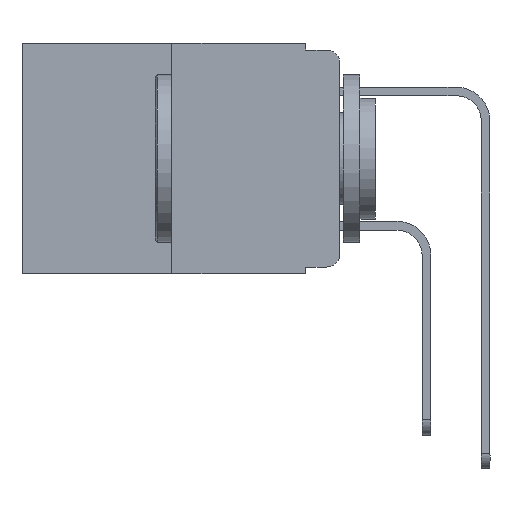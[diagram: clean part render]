
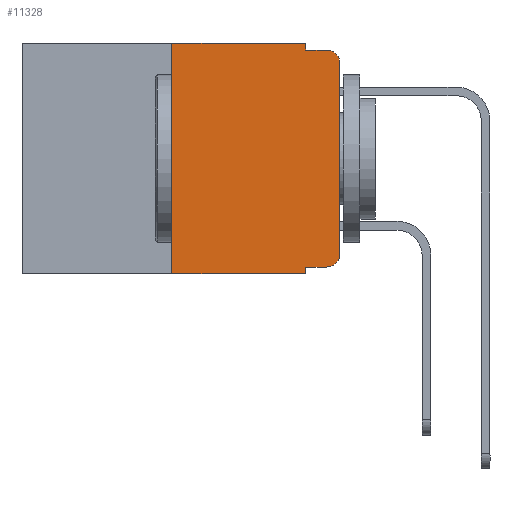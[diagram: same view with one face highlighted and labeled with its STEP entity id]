
A CAD part, left-side view. The second image highlights one B-rep face of the part: STEP entity #11328.
In plain terms, the highlighted planar face has unit normal (-1, 0, 0).
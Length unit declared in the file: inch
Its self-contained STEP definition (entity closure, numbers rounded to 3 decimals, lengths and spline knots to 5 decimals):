
#223 = AXIS2_PLACEMENT_3D ( 'NONE', #868, #13849, #3503 ) ;
#466 = EDGE_CURVE ( 'NONE', #8250, #16321, #9810, .T. ) ;
#662 = VERTEX_POINT ( 'NONE', #15351 ) ;
#868 = CARTESIAN_POINT ( 'NONE',  ( 0., 0.473, 0. ) ) ;
#1237 = DIRECTION ( 'NONE',  ( 0., 0., -1. ) ) ;
#1440 = VERTEX_POINT ( 'NONE', #16338 ) ;
#1577 = DIRECTION ( 'NONE',  ( 0., -1., 0. ) ) ;
#1847 = CARTESIAN_POINT ( 'NONE',  ( 0., 0.051, -0.343 ) ) ;
#1864 = CIRCLE ( 'NONE', #2945, 0.02 ) ;
#2131 = CARTESIAN_POINT ( 'NONE',  ( 0., 0., 0. ) ) ;
#2136 = VERTEX_POINT ( 'NONE', #7594 ) ;
#2229 = CARTESIAN_POINT ( 'NONE',  ( 0., 0.473, 0. ) ) ;
#2482 = DIRECTION ( 'NONE',  ( -1., 0., 0. ) ) ;
#2513 = CARTESIAN_POINT ( 'NONE',  ( 0., 0.02, -0.333 ) ) ;
#2811 = EDGE_CURVE ( 'NONE', #7481, #9059, #2869, .T. ) ;
#2869 = LINE ( 'NONE', #9188, #7181 ) ;
#2945 = AXIS2_PLACEMENT_3D ( 'NONE', #7443, #12659, #11380 ) ;
#3161 = VECTOR ( 'NONE', #6323, 39.37008 ) ;
#3177 = CARTESIAN_POINT ( 'NONE',  ( 0., 0.473, -0.343 ) ) ;
#3304 = ORIENTED_EDGE ( 'NONE', *, *, #466, .T. ) ;
#3503 = DIRECTION ( 'NONE',  ( 0., 0., -1. ) ) ;
#3561 = EDGE_CURVE ( 'NONE', #9451, #8250, #3597, .T. ) ;
#3597 = CIRCLE ( 'NONE', #4415, 0.02 ) ;
#3676 = PLANE ( 'NONE',  #223 ) ;
#3823 = VECTOR ( 'NONE', #1577, 39.37008 ) ;
#3964 = VECTOR ( 'NONE', #7245, 39.37008 ) ;
#4415 = AXIS2_PLACEMENT_3D ( 'NONE', #4936, #2482, #14090 ) ;
#4618 = VERTEX_POINT ( 'NONE', #13183 ) ;
#4823 = ORIENTED_EDGE ( 'NONE', *, *, #9868, .T. ) ;
#4837 = ORIENTED_EDGE ( 'NONE', *, *, #9538, .F. ) ;
#4936 = CARTESIAN_POINT ( 'NONE',  ( 0., 0.02, -0.313 ) ) ;
#4947 = EDGE_CURVE ( 'NONE', #1440, #2136, #16865, .T. ) ;
#5548 = ORIENTED_EDGE ( 'NONE', *, *, #2811, .F. ) ;
#6323 = DIRECTION ( 'NONE',  ( 0., -1., 0. ) ) ;
#7181 = VECTOR ( 'NONE', #12099, 39.37008 ) ;
#7245 = DIRECTION ( 'NONE',  ( 0., 0., 1. ) ) ;
#7443 = CARTESIAN_POINT ( 'NONE',  ( 0., 0.02, -0.03 ) ) ;
#7476 = CARTESIAN_POINT ( 'NONE',  ( 0., 0.051, -0.333 ) ) ;
#7481 = VERTEX_POINT ( 'NONE', #7476 ) ;
#7539 = VECTOR ( 'NONE', #11385, 39.37008 ) ;
#7594 = CARTESIAN_POINT ( 'NONE',  ( 0., 0.25, 0. ) ) ;
#8077 = ORIENTED_EDGE ( 'NONE', *, *, #11386, .T. ) ;
#8250 = VERTEX_POINT ( 'NONE', #14632 ) ;
#8394 = LINE ( 'NONE', #13427, #3823 ) ;
#8482 = VECTOR ( 'NONE', #14196, 39.37008 ) ;
#8981 = CARTESIAN_POINT ( 'NONE',  ( 0., 0.051, -0.333 ) ) ;
#9059 = VERTEX_POINT ( 'NONE', #1847 ) ;
#9102 = ORIENTED_EDGE ( 'NONE', *, *, #12095, .F. ) ;
#9188 = CARTESIAN_POINT ( 'NONE',  ( 0., 0.051, 0. ) ) ;
#9303 = VERTEX_POINT ( 'NONE', #15065 ) ;
#9451 = VERTEX_POINT ( 'NONE', #2513 ) ;
#9538 = EDGE_CURVE ( 'NONE', #662, #9303, #8394, .T. ) ;
#9810 = LINE ( 'NONE', #2131, #3964 ) ;
#9831 = ORIENTED_EDGE ( 'NONE', *, *, #14670, .T. ) ;
#9868 = EDGE_CURVE ( 'NONE', #7481, #9451, #10268, .T. ) ;
#10075 = LINE ( 'NONE', #2229, #3161 ) ;
#10268 = LINE ( 'NONE', #8981, #8482 ) ;
#10976 = ORIENTED_EDGE ( 'NONE', *, *, #3561, .T. ) ;
#11049 = DIRECTION ( 'NONE',  ( 0., -1., 0. ) ) ;
#11328 = ADVANCED_FACE ( 'NONE', ( #16510 ), #3676, .F. ) ;
#11380 = DIRECTION ( 'NONE',  ( 0., 0., -1. ) ) ;
#11385 = DIRECTION ( 'NONE',  ( 0., 0., 1. ) ) ;
#11386 = EDGE_CURVE ( 'NONE', #16321, #9303, #1864, .T. ) ;
#11579 = CARTESIAN_POINT ( 'NONE',  ( 0., 0., -0.03 ) ) ;
#11655 = CARTESIAN_POINT ( 'NONE',  ( 0., 0.051, 0. ) ) ;
#12095 = EDGE_CURVE ( 'NONE', #4618, #662, #15406, .T. ) ;
#12099 = DIRECTION ( 'NONE',  ( 0., 0., -1. ) ) ;
#12659 = DIRECTION ( 'NONE',  ( -1., 0., 0. ) ) ;
#13141 = VECTOR ( 'NONE', #1237, 39.37008 ) ;
#13183 = CARTESIAN_POINT ( 'NONE',  ( 0., 0.051, 0. ) ) ;
#13197 = ORIENTED_EDGE ( 'NONE', *, *, #16644, .F. ) ;
#13427 = CARTESIAN_POINT ( 'NONE',  ( 0., 0.051, -0.01 ) ) ;
#13849 = DIRECTION ( 'NONE',  ( 1., 0., 0. ) ) ;
#13944 = CARTESIAN_POINT ( 'NONE',  ( 0., 0.25, 0. ) ) ;
#14090 = DIRECTION ( 'NONE',  ( 0., 0., -1. ) ) ;
#14094 = ORIENTED_EDGE ( 'NONE', *, *, #4947, .F. ) ;
#14196 = DIRECTION ( 'NONE',  ( 0., -1., 0. ) ) ;
#14589 = VECTOR ( 'NONE', #11049, 39.37008 ) ;
#14632 = CARTESIAN_POINT ( 'NONE',  ( 0., 0., -0.313 ) ) ;
#14670 = EDGE_CURVE ( 'NONE', #1440, #9059, #14885, .T. ) ;
#14885 = LINE ( 'NONE', #3177, #14589 ) ;
#15065 = CARTESIAN_POINT ( 'NONE',  ( 0., 0.02, -0.01 ) ) ;
#15351 = CARTESIAN_POINT ( 'NONE',  ( 0., 0.051, -0.01 ) ) ;
#15406 = LINE ( 'NONE', #11655, #13141 ) ;
#16099 = EDGE_LOOP ( 'NONE', ( #3304, #8077, #4837, #9102, #13197, #14094, #9831, #5548, #4823, #10976 ) ) ;
#16321 = VERTEX_POINT ( 'NONE', #11579 ) ;
#16338 = CARTESIAN_POINT ( 'NONE',  ( 0., 0.25, -0.343 ) ) ;
#16510 = FACE_OUTER_BOUND ( 'NONE', #16099, .T. ) ;
#16644 = EDGE_CURVE ( 'NONE', #2136, #4618, #10075, .T. ) ;
#16865 = LINE ( 'NONE', #13944, #7539 ) ;
